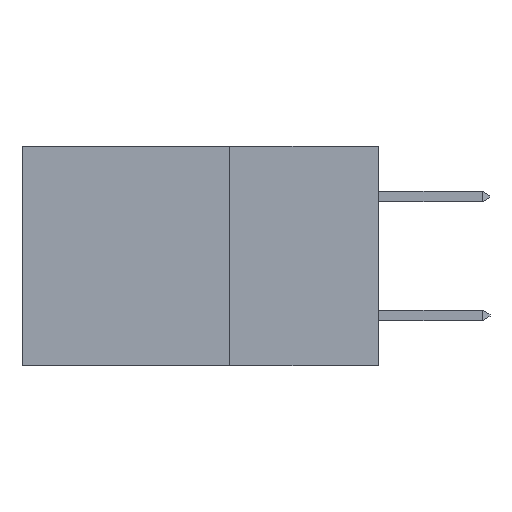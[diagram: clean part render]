
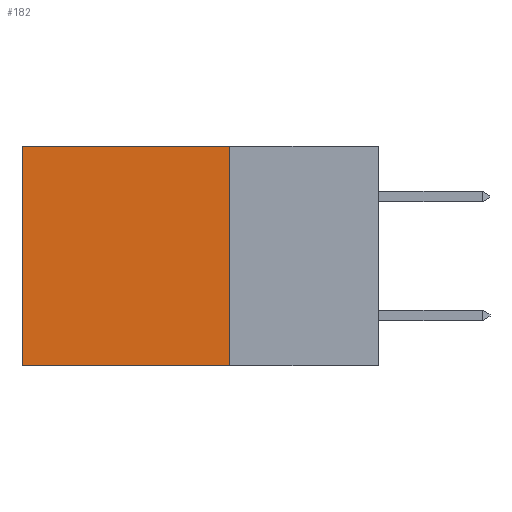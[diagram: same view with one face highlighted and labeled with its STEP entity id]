
A CAD part, left-side view. The second image highlights one B-rep face of the part: STEP entity #182.
In plain terms, the highlighted planar face has unit normal (-1, 0, 0).
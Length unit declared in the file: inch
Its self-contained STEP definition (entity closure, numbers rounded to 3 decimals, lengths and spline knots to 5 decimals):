
#134 = CARTESIAN_POINT ( 'NONE',  ( 0.2615, 0.25, -0.37 ) ) ;
#182 = ADVANCED_FACE ( 'NONE', ( #5932 ), #4041, .F. ) ;
#328 = VERTEX_POINT ( 'NONE', #134 ) ;
#478 = LINE ( 'NONE', #5057, #5745 ) ;
#561 = ORIENTED_EDGE ( 'NONE', *, *, #8067, .T. ) ;
#568 = DIRECTION ( 'NONE',  ( 0., 0., -1. ) ) ;
#670 = VECTOR ( 'NONE', #3987, 39.37008 ) ;
#931 = DIRECTION ( 'NONE',  ( 0., 1., 0. ) ) ;
#1666 = VERTEX_POINT ( 'NONE', #6481 ) ;
#1810 = EDGE_CURVE ( 'NONE', #1666, #328, #5421, .T. ) ;
#1828 = VECTOR ( 'NONE', #2879, 39.37008 ) ;
#2023 = VERTEX_POINT ( 'NONE', #7817 ) ;
#2879 = DIRECTION ( 'NONE',  ( 0., 0., -1. ) ) ;
#3017 = CARTESIAN_POINT ( 'NONE',  ( 0.2615, 0.25, -0.37 ) ) ;
#3218 = ORIENTED_EDGE ( 'NONE', *, *, #3255, .F. ) ;
#3255 = EDGE_CURVE ( 'NONE', #328, #2023, #6694, .T. ) ;
#3348 = ORIENTED_EDGE ( 'NONE', *, *, #3907, .T. ) ;
#3351 = AXIS2_PLACEMENT_3D ( 'NONE', #7445, #5118, #568 ) ;
#3907 = EDGE_CURVE ( 'NONE', #8018, #2023, #6304, .T. ) ;
#3968 = EDGE_LOOP ( 'NONE', ( #3348, #3218, #5838, #561 ) ) ;
#3987 = DIRECTION ( 'NONE',  ( 0., 0., -1. ) ) ;
#4018 = CARTESIAN_POINT ( 'NONE',  ( 0.2615, 0.6, -0.37 ) ) ;
#4041 = PLANE ( 'NONE',  #3351 ) ;
#5001 = VECTOR ( 'NONE', #6400, 39.37008 ) ;
#5057 = CARTESIAN_POINT ( 'NONE',  ( 0.2615, 0.25, 0. ) ) ;
#5118 = DIRECTION ( 'NONE',  ( 1., 0., 0. ) ) ;
#5421 = LINE ( 'NONE', #3017, #1828 ) ;
#5745 = VECTOR ( 'NONE', #931, 39.37008 ) ;
#5838 = ORIENTED_EDGE ( 'NONE', *, *, #1810, .F. ) ;
#5932 = FACE_OUTER_BOUND ( 'NONE', #3968, .T. ) ;
#6304 = LINE ( 'NONE', #4018, #670 ) ;
#6400 = DIRECTION ( 'NONE',  ( 0., 1., 0. ) ) ;
#6481 = CARTESIAN_POINT ( 'NONE',  ( 0.2615, 0.25, 0. ) ) ;
#6496 = CARTESIAN_POINT ( 'NONE',  ( 0.2615, 0.25, -0.37 ) ) ;
#6694 = LINE ( 'NONE', #6496, #5001 ) ;
#6922 = CARTESIAN_POINT ( 'NONE',  ( 0.2615, 0.6, 0. ) ) ;
#7445 = CARTESIAN_POINT ( 'NONE',  ( 0.2615, 0.25, -0.37 ) ) ;
#7817 = CARTESIAN_POINT ( 'NONE',  ( 0.2615, 0.6, -0.37 ) ) ;
#8018 = VERTEX_POINT ( 'NONE', #6922 ) ;
#8067 = EDGE_CURVE ( 'NONE', #1666, #8018, #478, .T. ) ;
